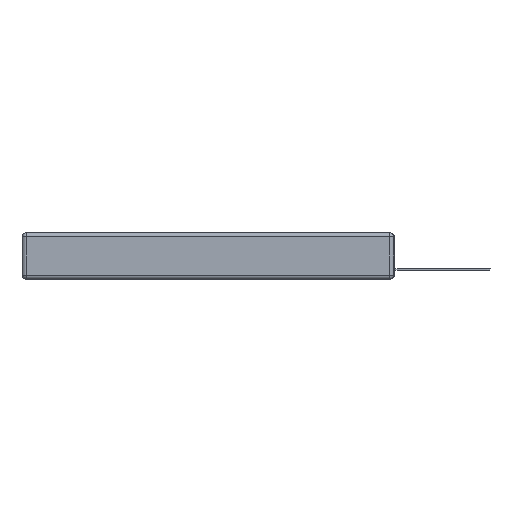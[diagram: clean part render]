
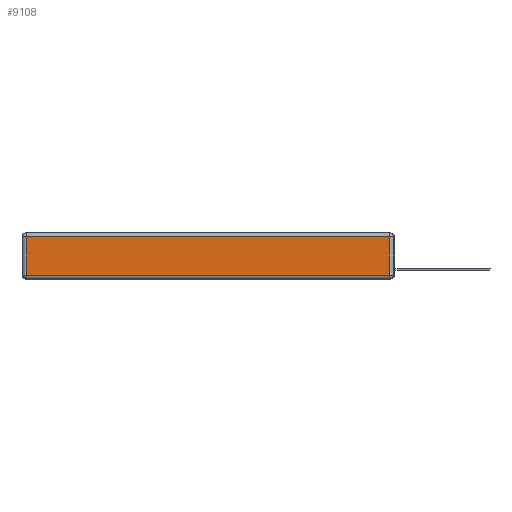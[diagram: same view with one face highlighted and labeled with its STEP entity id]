
A CAD part, left-side view. The second image highlights one B-rep face of the part: STEP entity #9108.
In plain terms, the highlighted planar face has unit normal (-1, 0, 0).
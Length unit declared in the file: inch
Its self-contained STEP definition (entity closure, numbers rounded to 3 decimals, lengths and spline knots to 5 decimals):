
#360 = DIRECTION ( 'NONE',  ( 0., -1., 0. ) ) ;
#988 = EDGE_CURVE ( 'NONE', #1778, #14142, #11713, .T. ) ;
#1065 = VECTOR ( 'NONE', #9587, 39.37008 ) ;
#1380 = EDGE_CURVE ( 'NONE', #6357, #12322, #4738, .T. ) ;
#1528 = LINE ( 'NONE', #11674, #3128 ) ;
#1778 = VERTEX_POINT ( 'NONE', #15113 ) ;
#3128 = VECTOR ( 'NONE', #360, 39.37008 ) ;
#3575 = CARTESIAN_POINT ( 'NONE',  ( 0., 2.72, -0.343 ) ) ;
#4738 = LINE ( 'NONE', #3575, #18075 ) ;
#4744 = PLANE ( 'NONE',  #5290 ) ;
#4837 = CARTESIAN_POINT ( 'NONE',  ( 0., 2.72, -0.03 ) ) ;
#4912 = FACE_OUTER_BOUND ( 'NONE', #5091, .T. ) ;
#5091 = EDGE_LOOP ( 'NONE', ( #5259, #18774, #5732, #16258 ) ) ;
#5259 = ORIENTED_EDGE ( 'NONE', *, *, #13036, .T. ) ;
#5290 = AXIS2_PLACEMENT_3D ( 'NONE', #7608, #14945, #15136 ) ;
#5732 = ORIENTED_EDGE ( 'NONE', *, *, #15320, .T. ) ;
#6342 = DIRECTION ( 'NONE',  ( 0., 0., -1. ) ) ;
#6357 = VERTEX_POINT ( 'NONE', #4837 ) ;
#7608 = CARTESIAN_POINT ( 'NONE',  ( 0., 0., -0.343 ) ) ;
#8765 = DIRECTION ( 'NONE',  ( 0., 0., 1. ) ) ;
#9108 = ADVANCED_FACE ( 'NONE', ( #4912 ), #4744, .T. ) ;
#9587 = DIRECTION ( 'NONE',  ( 0., 1., 0. ) ) ;
#9993 = CARTESIAN_POINT ( 'NONE',  ( 0., 0.03, -0.343 ) ) ;
#10928 = CARTESIAN_POINT ( 'NONE',  ( 0., 2.75, -0.03 ) ) ;
#11201 = CARTESIAN_POINT ( 'NONE',  ( 0., 0.03, -0.03 ) ) ;
#11674 = CARTESIAN_POINT ( 'NONE',  ( 0., 0., -0.313 ) ) ;
#11713 = LINE ( 'NONE', #9993, #14671 ) ;
#12322 = VERTEX_POINT ( 'NONE', #14082 ) ;
#13036 = EDGE_CURVE ( 'NONE', #12322, #1778, #1528, .T. ) ;
#14082 = CARTESIAN_POINT ( 'NONE',  ( 0., 2.72, -0.313 ) ) ;
#14142 = VERTEX_POINT ( 'NONE', #11201 ) ;
#14671 = VECTOR ( 'NONE', #8765, 39.37008 ) ;
#14945 = DIRECTION ( 'NONE',  ( -1., 0., 0. ) ) ;
#15113 = CARTESIAN_POINT ( 'NONE',  ( 0., 0.03, -0.313 ) ) ;
#15136 = DIRECTION ( 'NONE',  ( 0., 0., 1. ) ) ;
#15320 = EDGE_CURVE ( 'NONE', #14142, #6357, #18215, .T. ) ;
#16258 = ORIENTED_EDGE ( 'NONE', *, *, #1380, .T. ) ;
#18075 = VECTOR ( 'NONE', #6342, 39.37008 ) ;
#18215 = LINE ( 'NONE', #10928, #1065 ) ;
#18774 = ORIENTED_EDGE ( 'NONE', *, *, #988, .T. ) ;
